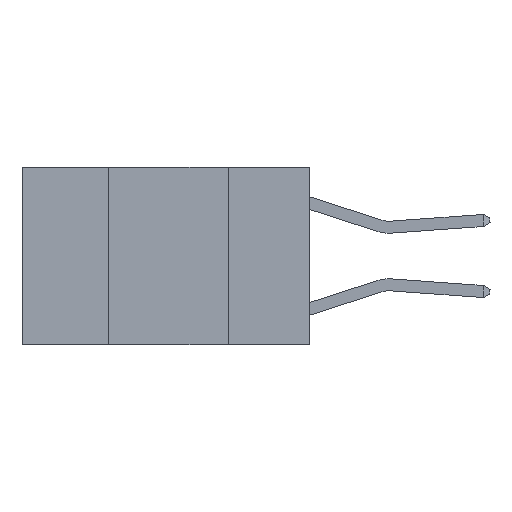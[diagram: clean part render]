
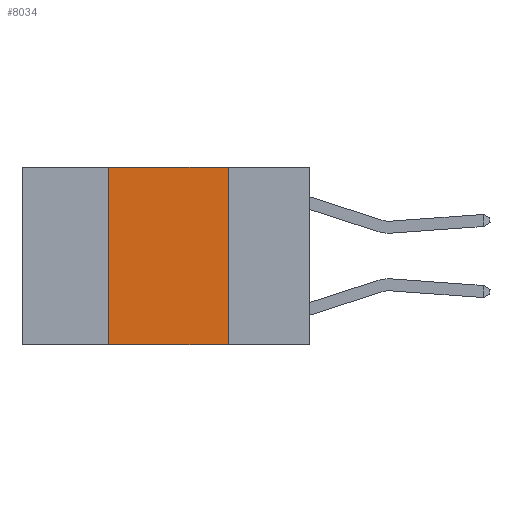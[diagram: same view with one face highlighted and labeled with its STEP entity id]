
A CAD part, left-side view. The second image highlights one B-rep face of the part: STEP entity #8034.
In plain terms, the highlighted planar face has unit normal (-1, 0, 0).
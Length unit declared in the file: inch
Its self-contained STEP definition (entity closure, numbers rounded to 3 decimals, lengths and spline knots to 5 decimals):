
#130 = EDGE_CURVE ( 'NONE', #9697, #5427, #1693, .T. ) ;
#213 = DIRECTION ( 'NONE',  ( 1., 0., 0. ) ) ;
#790 = CARTESIAN_POINT ( 'NONE',  ( 0., 0.17, 0. ) ) ;
#1159 = CARTESIAN_POINT ( 'NONE',  ( 0., 0.42, -0.37 ) ) ;
#1192 = EDGE_CURVE ( 'NONE', #2904, #10619, #1701, .T. ) ;
#1546 = ORIENTED_EDGE ( 'NONE', *, *, #7330, .T. ) ;
#1693 = LINE ( 'NONE', #7150, #3568 ) ;
#1694 = VECTOR ( 'NONE', #4712, 39.37008 ) ;
#1701 = LINE ( 'NONE', #790, #10582 ) ;
#1835 = LINE ( 'NONE', #6616, #1694 ) ;
#1944 = FACE_OUTER_BOUND ( 'NONE', #10812, .T. ) ;
#2730 = DIRECTION ( 'NONE',  ( 0., 0., -1. ) ) ;
#2904 = VERTEX_POINT ( 'NONE', #7190 ) ;
#3153 = CARTESIAN_POINT ( 'NONE',  ( 0., 0.42, 0. ) ) ;
#3532 = DIRECTION ( 'NONE',  ( 0., 0., 1. ) ) ;
#3568 = VECTOR ( 'NONE', #3532, 39.37008 ) ;
#4017 = DIRECTION ( 'NONE',  ( 0., -1., 0. ) ) ;
#4287 = VECTOR ( 'NONE', #4017, 39.37008 ) ;
#4712 = DIRECTION ( 'NONE',  ( 0., -1., 0. ) ) ;
#4953 = LINE ( 'NONE', #8689, #4287 ) ;
#5278 = AXIS2_PLACEMENT_3D ( 'NONE', #8521, #213, #11491 ) ;
#5400 = CARTESIAN_POINT ( 'NONE',  ( 0., 0.17, -0.37 ) ) ;
#5427 = VERTEX_POINT ( 'NONE', #3153 ) ;
#5840 = ORIENTED_EDGE ( 'NONE', *, *, #1192, .F. ) ;
#6435 = ORIENTED_EDGE ( 'NONE', *, *, #6519, .F. ) ;
#6519 = EDGE_CURVE ( 'NONE', #5427, #2904, #1835, .T. ) ;
#6616 = CARTESIAN_POINT ( 'NONE',  ( 0., 0.6, 0. ) ) ;
#7150 = CARTESIAN_POINT ( 'NONE',  ( 0., 0.42, 0. ) ) ;
#7190 = CARTESIAN_POINT ( 'NONE',  ( 0., 0.17, 0. ) ) ;
#7330 = EDGE_CURVE ( 'NONE', #9697, #10619, #4953, .T. ) ;
#8034 = ADVANCED_FACE ( 'NONE', ( #1944 ), #8674, .F. ) ;
#8521 = CARTESIAN_POINT ( 'NONE',  ( 0., 0.6, 0. ) ) ;
#8674 = PLANE ( 'NONE',  #5278 ) ;
#8689 = CARTESIAN_POINT ( 'NONE',  ( 0., 0.6, -0.37 ) ) ;
#9697 = VERTEX_POINT ( 'NONE', #1159 ) ;
#10582 = VECTOR ( 'NONE', #2730, 39.37008 ) ;
#10619 = VERTEX_POINT ( 'NONE', #5400 ) ;
#10812 = EDGE_LOOP ( 'NONE', ( #5840, #6435, #10977, #1546 ) ) ;
#10977 = ORIENTED_EDGE ( 'NONE', *, *, #130, .F. ) ;
#11491 = DIRECTION ( 'NONE',  ( 0., 0., -1. ) ) ;
